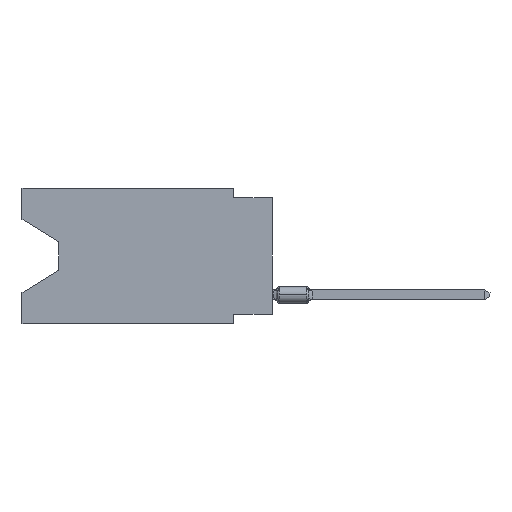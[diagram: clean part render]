
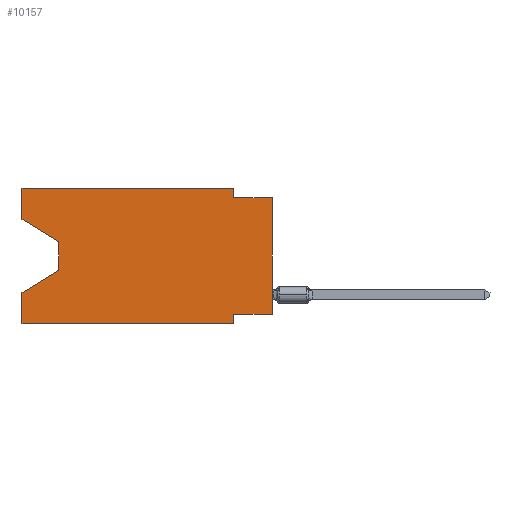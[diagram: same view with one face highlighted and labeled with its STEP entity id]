
A CAD part, left-side view. The second image highlights one B-rep face of the part: STEP entity #10157.
In plain terms, the highlighted planar face has unit normal (-1, 0, 0).
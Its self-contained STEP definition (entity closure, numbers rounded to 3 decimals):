
#43 = LINE ( 'NONE', #1625, #3293 ) ;
#60 = DIRECTION ( 'NONE',  ( 0., 0., 1. ) ) ;
#190 = ORIENTED_EDGE ( 'NONE', *, *, #11365, .T. ) ;
#389 = CARTESIAN_POINT ( 'NONE',  ( 0., 2.54, -8.89 ) ) ;
#409 = CARTESIAN_POINT ( 'NONE',  ( 0., 0., -8.255 ) ) ;
#874 = VERTEX_POINT ( 'NONE', #409 ) ;
#1625 = CARTESIAN_POINT ( 'NONE',  ( 0., 2.54, 0. ) ) ;
#1628 = ORIENTED_EDGE ( 'NONE', *, *, #11542, .F. ) ;
#2142 = DIRECTION ( 'NONE',  ( 0., -1., 0. ) ) ;
#2315 = VERTEX_POINT ( 'NONE', #14207 ) ;
#2577 = VERTEX_POINT ( 'NONE', #22158 ) ;
#3009 = CARTESIAN_POINT ( 'NONE',  ( 0., 13.97, -3.505 ) ) ;
#3293 = VECTOR ( 'NONE', #8548, 1000. ) ;
#3405 = VECTOR ( 'NONE', #21547, 1000. ) ;
#3692 = DIRECTION ( 'NONE',  ( 0., 0., 1. ) ) ;
#3749 = CARTESIAN_POINT ( 'NONE',  ( 0., 16.383, -6.852 ) ) ;
#3969 = LINE ( 'NONE', #12465, #11940 ) ;
#3978 = DIRECTION ( 'NONE',  ( 0., -1., 0. ) ) ;
#4006 = VECTOR ( 'NONE', #9682, 1000. ) ;
#4025 = LINE ( 'NONE', #3009, #4006 ) ;
#4160 = VERTEX_POINT ( 'NONE', #7607 ) ;
#4390 = LINE ( 'NONE', #21737, #7166 ) ;
#4486 = ORIENTED_EDGE ( 'NONE', *, *, #20743, .T. ) ;
#4497 = VECTOR ( 'NONE', #5321, 1000. ) ;
#4507 = CARTESIAN_POINT ( 'NONE',  ( 0., 16.383, -8.89 ) ) ;
#4709 = VERTEX_POINT ( 'NONE', #14180 ) ;
#5082 = VECTOR ( 'NONE', #14570, 1000. ) ;
#5321 = DIRECTION ( 'NONE',  ( 0., 0.855, -0.519 ) ) ;
#5556 = AXIS2_PLACEMENT_3D ( 'NONE', #18534, #20004, #15230 ) ;
#5624 = ORIENTED_EDGE ( 'NONE', *, *, #7842, .T. ) ;
#5718 = LINE ( 'NONE', #7188, #20724 ) ;
#5822 = ORIENTED_EDGE ( 'NONE', *, *, #19978, .F. ) ;
#5974 = ORIENTED_EDGE ( 'NONE', *, *, #13153, .F. ) ;
#6212 = LINE ( 'NONE', #20057, #8102 ) ;
#7166 = VECTOR ( 'NONE', #8135, 1000. ) ;
#7188 = CARTESIAN_POINT ( 'NONE',  ( 0., 16.383, 0. ) ) ;
#7291 = EDGE_CURVE ( 'NONE', #2577, #8075, #14507, .T. ) ;
#7441 = CARTESIAN_POINT ( 'NONE',  ( 0., 16.383, -2.038 ) ) ;
#7607 = CARTESIAN_POINT ( 'NONE',  ( 0., 13.97, -3.505 ) ) ;
#7821 = CARTESIAN_POINT ( 'NONE',  ( 0., 16.383, 0. ) ) ;
#7842 = EDGE_CURVE ( 'NONE', #874, #15215, #6212, .T. ) ;
#8046 = EDGE_CURVE ( 'NONE', #874, #22065, #18250, .T. ) ;
#8075 = VERTEX_POINT ( 'NONE', #13034 ) ;
#8102 = VECTOR ( 'NONE', #60, 1000. ) ;
#8135 = DIRECTION ( 'NONE',  ( 0., -1., 0. ) ) ;
#8321 = PLANE ( 'NONE',  #5556 ) ;
#8548 = DIRECTION ( 'NONE',  ( 0., 0., -1. ) ) ;
#8859 = CARTESIAN_POINT ( 'NONE',  ( 0., 2.54, -8.255 ) ) ;
#9164 = VECTOR ( 'NONE', #21616, 1000. ) ;
#9682 = DIRECTION ( 'NONE',  ( 0., 0., -1. ) ) ;
#10157 = ADVANCED_FACE ( 'NONE', ( #16829 ), #8321, .F. ) ;
#10710 = EDGE_CURVE ( 'NONE', #2315, #20793, #12330, .T. ) ;
#11221 = CARTESIAN_POINT ( 'NONE',  ( 0., 0., -8.255 ) ) ;
#11365 = EDGE_CURVE ( 'NONE', #4160, #2315, #4025, .T. ) ;
#11542 = EDGE_CURVE ( 'NONE', #8075, #4709, #43, .T. ) ;
#11940 = VECTOR ( 'NONE', #2142, 1000. ) ;
#11993 = EDGE_LOOP ( 'NONE', ( #15624, #190, #18015, #13257, #4486, #21928, #15275, #5624, #5822, #1628, #16718, #5974 ) ) ;
#12330 = LINE ( 'NONE', #14028, #4497 ) ;
#12465 = CARTESIAN_POINT ( 'NONE',  ( 0., 16.383, -8.89 ) ) ;
#13034 = CARTESIAN_POINT ( 'NONE',  ( 0., 2.54, 0. ) ) ;
#13153 = EDGE_CURVE ( 'NONE', #22211, #2577, #5718, .T. ) ;
#13155 = VECTOR ( 'NONE', #3978, 1000. ) ;
#13257 = ORIENTED_EDGE ( 'NONE', *, *, #16083, .F. ) ;
#14028 = CARTESIAN_POINT ( 'NONE',  ( 0., 13.97, -5.385 ) ) ;
#14180 = CARTESIAN_POINT ( 'NONE',  ( 0., 2.54, -0.635 ) ) ;
#14207 = CARTESIAN_POINT ( 'NONE',  ( 0., 13.97, -5.385 ) ) ;
#14284 = EDGE_CURVE ( 'NONE', #22211, #4160, #14691, .T. ) ;
#14507 = LINE ( 'NONE', #7821, #13155 ) ;
#14570 = DIRECTION ( 'NONE',  ( 0., 0., -1. ) ) ;
#14691 = LINE ( 'NONE', #7441, #9164 ) ;
#14804 = VECTOR ( 'NONE', #21322, 1000. ) ;
#15215 = VERTEX_POINT ( 'NONE', #20870 ) ;
#15230 = DIRECTION ( 'NONE',  ( 0., 0., -1. ) ) ;
#15275 = ORIENTED_EDGE ( 'NONE', *, *, #8046, .F. ) ;
#15624 = ORIENTED_EDGE ( 'NONE', *, *, #14284, .T. ) ;
#15934 = LINE ( 'NONE', #19678, #5082 ) ;
#16083 = EDGE_CURVE ( 'NONE', #20018, #20793, #21667, .T. ) ;
#16718 = ORIENTED_EDGE ( 'NONE', *, *, #7291, .F. ) ;
#16829 = FACE_OUTER_BOUND ( 'NONE', #11993, .T. ) ;
#18015 = ORIENTED_EDGE ( 'NONE', *, *, #10710, .T. ) ;
#18250 = LINE ( 'NONE', #11221, #3405 ) ;
#18258 = CARTESIAN_POINT ( 'NONE',  ( 0., 16.383, 0. ) ) ;
#18534 = CARTESIAN_POINT ( 'NONE',  ( 0., 16.383, 0. ) ) ;
#18664 = VERTEX_POINT ( 'NONE', #389 ) ;
#19678 = CARTESIAN_POINT ( 'NONE',  ( 0., 2.54, -8.89 ) ) ;
#19978 = EDGE_CURVE ( 'NONE', #4709, #15215, #4390, .T. ) ;
#20004 = DIRECTION ( 'NONE',  ( 1., 0., 0. ) ) ;
#20018 = VERTEX_POINT ( 'NONE', #4507 ) ;
#20057 = CARTESIAN_POINT ( 'NONE',  ( 0., 0., 0. ) ) ;
#20724 = VECTOR ( 'NONE', #3692, 1000. ) ;
#20743 = EDGE_CURVE ( 'NONE', #20018, #18664, #3969, .T. ) ;
#20793 = VERTEX_POINT ( 'NONE', #3749 ) ;
#20870 = CARTESIAN_POINT ( 'NONE',  ( 0., 0., -0.635 ) ) ;
#20975 = EDGE_CURVE ( 'NONE', #22065, #18664, #15934, .T. ) ;
#21322 = DIRECTION ( 'NONE',  ( 0., 0., 1. ) ) ;
#21440 = CARTESIAN_POINT ( 'NONE',  ( 0., 16.383, -2.038 ) ) ;
#21547 = DIRECTION ( 'NONE',  ( 0., 1., 0. ) ) ;
#21616 = DIRECTION ( 'NONE',  ( 0., -0.855, -0.519 ) ) ;
#21667 = LINE ( 'NONE', #18258, #14804 ) ;
#21737 = CARTESIAN_POINT ( 'NONE',  ( 0., 0., -0.635 ) ) ;
#21928 = ORIENTED_EDGE ( 'NONE', *, *, #20975, .F. ) ;
#22065 = VERTEX_POINT ( 'NONE', #8859 ) ;
#22158 = CARTESIAN_POINT ( 'NONE',  ( 0., 16.383, 0. ) ) ;
#22211 = VERTEX_POINT ( 'NONE', #21440 ) ;
